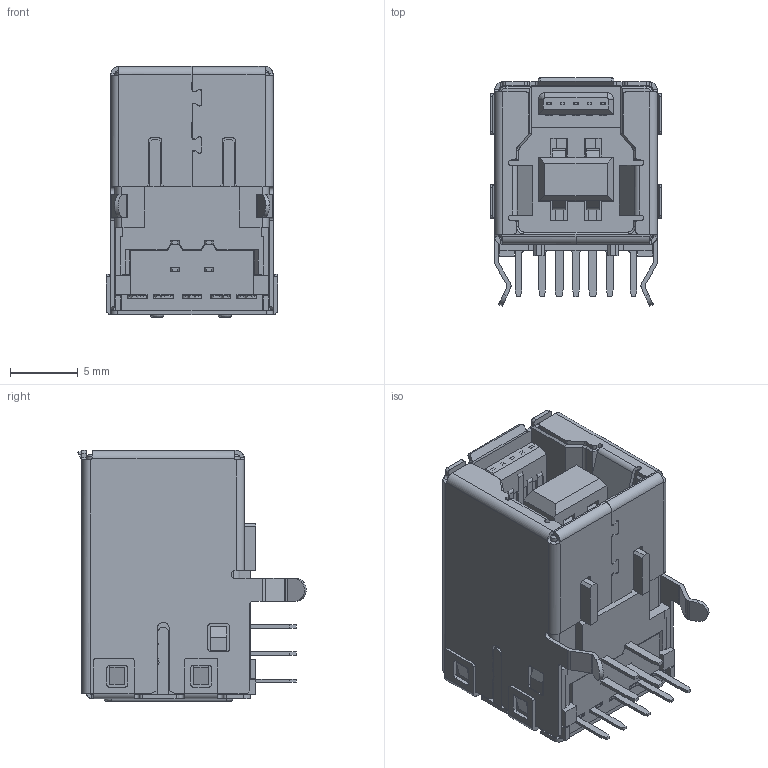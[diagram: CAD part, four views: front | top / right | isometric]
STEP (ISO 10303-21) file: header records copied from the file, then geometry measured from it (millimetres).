
FILE_DESCRIPTION (( 'STEP AP214' ), '1' );
FILE_NAME ('690P209-12C-022.STEP', '2021-01-14T21:04:00', ( '' ), ( '' ), 'SwSTEP 2.0', 'SolidWorks 2020', '' );
FILE_SCHEMA (( 'AUTOMOTIVE_DESIGN' ));
Length unit declared in the file: millimetre
Products named in the file (13): Contact2 690P209-X2C-02X; Insulator1 690P209-X2C-02X_Blue; Contact6 690P209-X2C-02X; Shell2 690P209-X2C-02X; Contact7 690P209-X2C-02X; Shell 690P209-X2C-02X; Insulator3 690P209-X2C-02X_Blue; 690P209-12C-022; Contact5 690P209-X2C-02X; Contact1 690P209-X2C-02X; Contact9 690P209-X2C-02X; Insulator2 690P209-X2C-02X_Blue; Contact8 690P209-X2C-02X
Assembly tree (14 placements, depth 2):
  690P209-12C-022
    Shell 690P209-X2C-02X
    Insulator1 690P209-X2C-02X_Blue
    Contact7 690P209-X2C-02X
    Insulator2 690P209-X2C-02X_Blue
    Contact6 690P209-X2C-02X
    Contact5 690P209-X2C-02X
    Contact8 690P209-X2C-02X
    Contact9 690P209-X2C-02X
    Insulator3 690P209-X2C-02X_Blue
    Shell2 690P209-X2C-02X
    Contact1 690P209-X2C-02X  x2
    Contact2 690P209-X2C-02X  x2
Bounding box: 12.7 x 16.88 x 18.55 mm (x, y, z)
Volume: 1478.6 mm3; surface area: 5371.6 mm2
Topology: 14 solids, 14 shells, 1485 faces, 4155 edges, 2702 vertices
Faces by surface type: plane 1057, cylinder 354, bspline 60, cone 14
Entity records: 46199 total; most frequent: CARTESIAN_POINT 11474, ORIENTED_EDGE 7528, DIRECTION 6455, EDGE_CURVE 3764, VECTOR 2969, LINE 2969, VERTEX_POINT 2444, AXIS2_PLACEMENT_3D 1743
